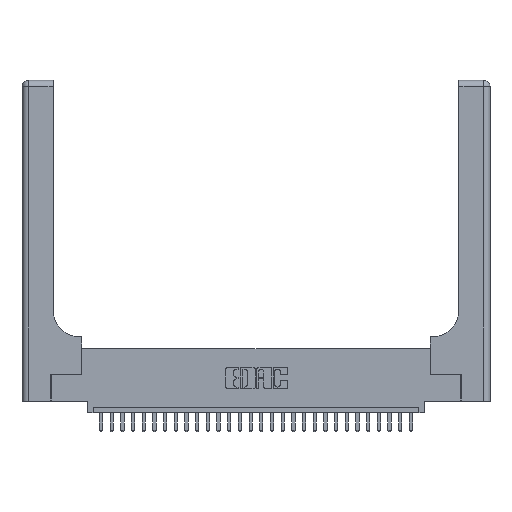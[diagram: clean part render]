
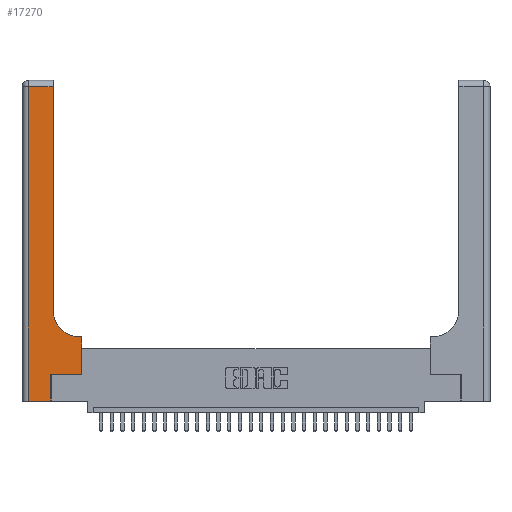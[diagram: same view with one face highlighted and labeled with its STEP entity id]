
A CAD part, top view. The second image highlights one B-rep face of the part: STEP entity #17270.
In plain terms, the highlighted planar face has unit normal (0, 0, 1).
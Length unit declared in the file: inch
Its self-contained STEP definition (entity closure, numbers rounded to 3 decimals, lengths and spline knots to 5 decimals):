
#616 = CARTESIAN_POINT ( 'NONE',  ( 0.269, 0., 0.37 ) ) ;
#768 = VECTOR ( 'NONE', #22380, 39.37008 ) ;
#1608 = EDGE_CURVE ( 'NONE', #26758, #4401, #22661, .T. ) ;
#1623 = DIRECTION ( 'NONE',  ( 0., 0., -1. ) ) ;
#1787 = CARTESIAN_POINT ( 'NONE',  ( 0.2915, 2.94, 0.37 ) ) ;
#2602 = VERTEX_POINT ( 'NONE', #6383 ) ;
#2811 = DIRECTION ( 'NONE',  ( 0., -1., 0. ) ) ;
#3104 = VECTOR ( 'NONE', #2811, 39.37008 ) ;
#3581 = DIRECTION ( 'NONE',  ( 1., 0., 0. ) ) ;
#3764 = EDGE_CURVE ( 'NONE', #22799, #18653, #8235, .T. ) ;
#3940 = DIRECTION ( 'NONE',  ( -1., 0., 0. ) ) ;
#3974 = DIRECTION ( 'NONE',  ( 1., 0., 0. ) ) ;
#4401 = VERTEX_POINT ( 'NONE', #616 ) ;
#4444 = LINE ( 'NONE', #28462, #17670 ) ;
#4552 = CARTESIAN_POINT ( 'NONE',  ( 0.2915, 3., 0.37 ) ) ;
#5438 = VERTEX_POINT ( 'NONE', #21865 ) ;
#6383 = CARTESIAN_POINT ( 'NONE',  ( 0.5585, 0.25, 0.37 ) ) ;
#7422 = LINE ( 'NONE', #10537, #23918 ) ;
#7733 = EDGE_CURVE ( 'NONE', #2602, #22799, #19008, .T. ) ;
#7748 = CIRCLE ( 'NONE', #20116, 0.25 ) ;
#7822 = EDGE_CURVE ( 'NONE', #4401, #23306, #15807, .T. ) ;
#8235 = LINE ( 'NONE', #19812, #23263 ) ;
#8492 = PLANE ( 'NONE',  #10880 ) ;
#8496 = DIRECTION ( 'NONE',  ( -1., 0., 0. ) ) ;
#8664 = CARTESIAN_POINT ( 'NONE',  ( 0.269, 0.25, 0.37 ) ) ;
#9491 = EDGE_CURVE ( 'NONE', #18653, #5438, #7748, .T. ) ;
#9619 = ORIENTED_EDGE ( 'NONE', *, *, #9491, .T. ) ;
#9697 = VECTOR ( 'NONE', #13705, 39.37008 ) ;
#9846 = EDGE_CURVE ( 'NONE', #11916, #26758, #10611, .T. ) ;
#10467 = CARTESIAN_POINT ( 'NONE',  ( 0.06, 3., 0.37 ) ) ;
#10537 = CARTESIAN_POINT ( 'NONE',  ( 0.269, 0.25, 0.37 ) ) ;
#10611 = LINE ( 'NONE', #10467, #3104 ) ;
#10880 = AXIS2_PLACEMENT_3D ( 'NONE', #29008, #1623, #3940 ) ;
#11622 = FACE_OUTER_BOUND ( 'NONE', #25644, .T. ) ;
#11916 = VERTEX_POINT ( 'NONE', #18664 ) ;
#12825 = CARTESIAN_POINT ( 'NONE',  ( 0.06, 0., 0.37 ) ) ;
#13058 = ORIENTED_EDGE ( 'NONE', *, *, #3764, .T. ) ;
#13705 = DIRECTION ( 'NONE',  ( 0., 1., 0. ) ) ;
#13779 = LINE ( 'NONE', #4552, #23440 ) ;
#14925 = CARTESIAN_POINT ( 'NONE',  ( 0.5415, 0.85, 0.37 ) ) ;
#15460 = CARTESIAN_POINT ( 'NONE',  ( 0.5585, 0.25, 0.37 ) ) ;
#15807 = LINE ( 'NONE', #20539, #9697 ) ;
#16228 = ORIENTED_EDGE ( 'NONE', *, *, #1608, .T. ) ;
#17136 = DIRECTION ( 'NONE',  ( 1., 0., 0. ) ) ;
#17270 = ADVANCED_FACE ( 'NONE', ( #11622 ), #8492, .F. ) ;
#17670 = VECTOR ( 'NONE', #19560, 39.37008 ) ;
#18052 = DIRECTION ( 'NONE',  ( 0., 1., 0. ) ) ;
#18056 = VERTEX_POINT ( 'NONE', #1787 ) ;
#18653 = VERTEX_POINT ( 'NONE', #23646 ) ;
#18664 = CARTESIAN_POINT ( 'NONE',  ( 0.06, 2.94, 0.37 ) ) ;
#18696 = VECTOR ( 'NONE', #3581, 39.37008 ) ;
#19008 = LINE ( 'NONE', #15460, #768 ) ;
#19560 = DIRECTION ( 'NONE',  ( -1., 0., 0. ) ) ;
#19812 = CARTESIAN_POINT ( 'NONE',  ( 0.2915, 0.6, 0.37 ) ) ;
#20116 = AXIS2_PLACEMENT_3D ( 'NONE', #14925, #26046, #17136 ) ;
#20539 = CARTESIAN_POINT ( 'NONE',  ( 0.269, 0., 0.37 ) ) ;
#21865 = CARTESIAN_POINT ( 'NONE',  ( 0.2915, 0.85, 0.37 ) ) ;
#22380 = DIRECTION ( 'NONE',  ( 0., 1., 0. ) ) ;
#22382 = EDGE_CURVE ( 'NONE', #18056, #11916, #4444, .T. ) ;
#22661 = LINE ( 'NONE', #25959, #18696 ) ;
#22799 = VERTEX_POINT ( 'NONE', #25333 ) ;
#23263 = VECTOR ( 'NONE', #8496, 39.37008 ) ;
#23306 = VERTEX_POINT ( 'NONE', #8664 ) ;
#23440 = VECTOR ( 'NONE', #18052, 39.37008 ) ;
#23646 = CARTESIAN_POINT ( 'NONE',  ( 0.5415, 0.6, 0.37 ) ) ;
#23866 = ORIENTED_EDGE ( 'NONE', *, *, #9846, .T. ) ;
#23918 = VECTOR ( 'NONE', #3974, 39.37008 ) ;
#24067 = ORIENTED_EDGE ( 'NONE', *, *, #27063, .T. ) ;
#25333 = CARTESIAN_POINT ( 'NONE',  ( 0.5585, 0.6, 0.37 ) ) ;
#25581 = EDGE_CURVE ( 'NONE', #23306, #2602, #7422, .T. ) ;
#25644 = EDGE_LOOP ( 'NONE', ( #24067, #27275, #23866, #16228, #27687, #28984, #29516, #13058, #9619 ) ) ;
#25959 = CARTESIAN_POINT ( 'NONE',  ( 0., 0., 0.37 ) ) ;
#26046 = DIRECTION ( 'NONE',  ( 0., 0., -1. ) ) ;
#26758 = VERTEX_POINT ( 'NONE', #12825 ) ;
#27063 = EDGE_CURVE ( 'NONE', #5438, #18056, #13779, .T. ) ;
#27275 = ORIENTED_EDGE ( 'NONE', *, *, #22382, .T. ) ;
#27687 = ORIENTED_EDGE ( 'NONE', *, *, #7822, .T. ) ;
#28462 = CARTESIAN_POINT ( 'NONE',  ( 0., 2.94, 0.37 ) ) ;
#28984 = ORIENTED_EDGE ( 'NONE', *, *, #25581, .T. ) ;
#29008 = CARTESIAN_POINT ( 'NONE',  ( 0., 3., 0.37 ) ) ;
#29516 = ORIENTED_EDGE ( 'NONE', *, *, #7733, .T. ) ;
